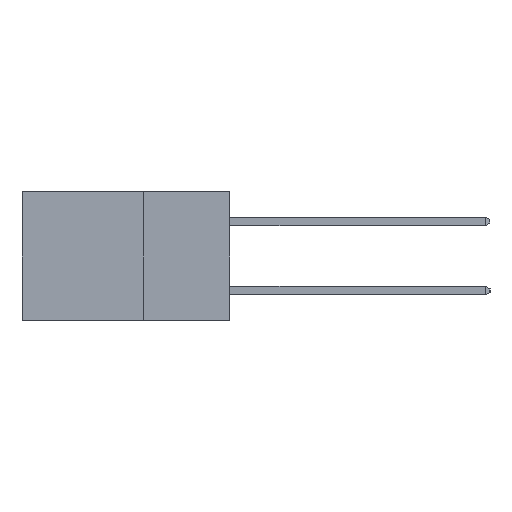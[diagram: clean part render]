
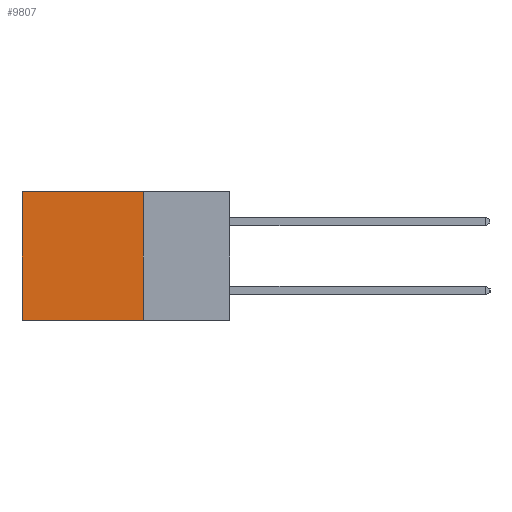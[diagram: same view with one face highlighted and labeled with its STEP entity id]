
A CAD part, left-side view. The second image highlights one B-rep face of the part: STEP entity #9807.
In plain terms, the highlighted planar face has unit normal (-1, 0, 0).
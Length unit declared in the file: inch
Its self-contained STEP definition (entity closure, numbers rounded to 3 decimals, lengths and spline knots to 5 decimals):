
#220 = DIRECTION ( 'NONE',  ( 0., 0., -1. ) ) ;
#285 = VERTEX_POINT ( 'NONE', #5049 ) ;
#640 = DIRECTION ( 'NONE',  ( 0., 1., 0. ) ) ;
#670 = CARTESIAN_POINT ( 'NONE',  ( 0.2615, 0.25, -0.37 ) ) ;
#1342 = VECTOR ( 'NONE', #3679, 39.37008 ) ;
#2328 = CARTESIAN_POINT ( 'NONE',  ( 0.2615, 0.25, 0. ) ) ;
#3679 = DIRECTION ( 'NONE',  ( 0., 0., -1. ) ) ;
#4026 = CARTESIAN_POINT ( 'NONE',  ( 0.2615, 0.25, 0. ) ) ;
#4056 = EDGE_CURVE ( 'NONE', #11810, #285, #13415, .T. ) ;
#4068 = ORIENTED_EDGE ( 'NONE', *, *, #4702, .T. ) ;
#4420 = CARTESIAN_POINT ( 'NONE',  ( 0.2615, 0.6, 0. ) ) ;
#4437 = CARTESIAN_POINT ( 'NONE',  ( 0.2615, 0.6, -0.37 ) ) ;
#4677 = DIRECTION ( 'NONE',  ( 0., 1., 0. ) ) ;
#4702 = EDGE_CURVE ( 'NONE', #5666, #11810, #10794, .T. ) ;
#5049 = CARTESIAN_POINT ( 'NONE',  ( 0.2615, 0.6, -0.37 ) ) ;
#5491 = LINE ( 'NONE', #9086, #8240 ) ;
#5657 = CARTESIAN_POINT ( 'NONE',  ( 0.2615, 0.25, -0.37 ) ) ;
#5666 = VERTEX_POINT ( 'NONE', #4026 ) ;
#6247 = EDGE_LOOP ( 'NONE', ( #14128, #9050, #11623, #4068 ) ) ;
#7007 = VECTOR ( 'NONE', #4677, 39.37008 ) ;
#7127 = LINE ( 'NONE', #670, #9833 ) ;
#7343 = DIRECTION ( 'NONE',  ( 1., 0., 0. ) ) ;
#7508 = EDGE_CURVE ( 'NONE', #7696, #285, #7127, .T. ) ;
#7696 = VERTEX_POINT ( 'NONE', #5657 ) ;
#8240 = VECTOR ( 'NONE', #10215, 39.37008 ) ;
#8706 = FACE_OUTER_BOUND ( 'NONE', #6247, .T. ) ;
#9050 = ORIENTED_EDGE ( 'NONE', *, *, #7508, .F. ) ;
#9086 = CARTESIAN_POINT ( 'NONE',  ( 0.2615, 0.25, -0.37 ) ) ;
#9807 = ADVANCED_FACE ( 'NONE', ( #8706 ), #11902, .F. ) ;
#9833 = VECTOR ( 'NONE', #640, 39.37008 ) ;
#10215 = DIRECTION ( 'NONE',  ( 0., 0., -1. ) ) ;
#10794 = LINE ( 'NONE', #2328, #7007 ) ;
#11279 = EDGE_CURVE ( 'NONE', #5666, #7696, #5491, .T. ) ;
#11623 = ORIENTED_EDGE ( 'NONE', *, *, #11279, .F. ) ;
#11810 = VERTEX_POINT ( 'NONE', #4420 ) ;
#11902 = PLANE ( 'NONE',  #12083 ) ;
#12083 = AXIS2_PLACEMENT_3D ( 'NONE', #13059, #7343, #220 ) ;
#13059 = CARTESIAN_POINT ( 'NONE',  ( 0.2615, 0.25, -0.37 ) ) ;
#13415 = LINE ( 'NONE', #4437, #1342 ) ;
#14128 = ORIENTED_EDGE ( 'NONE', *, *, #4056, .T. ) ;
